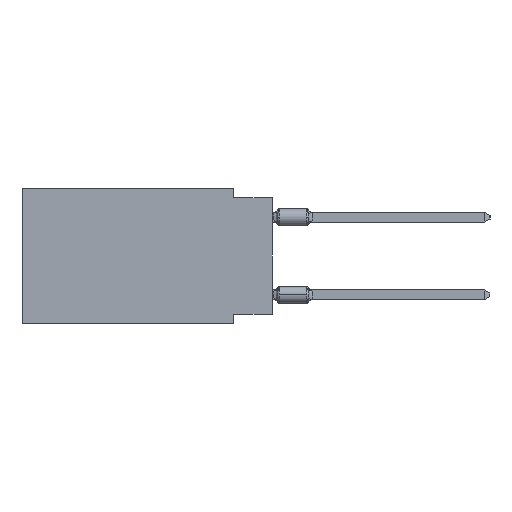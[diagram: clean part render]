
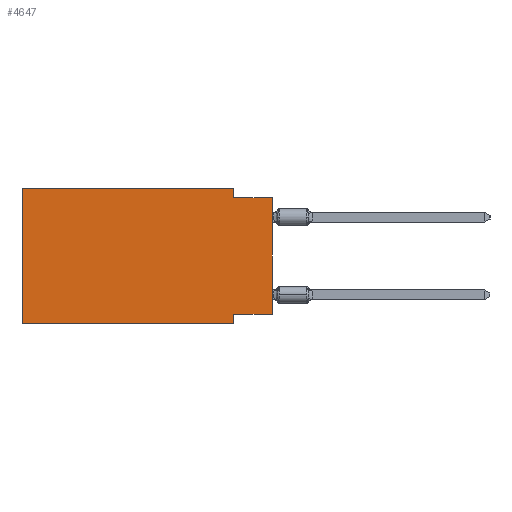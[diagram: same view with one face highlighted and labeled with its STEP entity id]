
A CAD part, left-side view. The second image highlights one B-rep face of the part: STEP entity #4647.
In plain terms, the highlighted planar face has unit normal (-1, 0, 0).
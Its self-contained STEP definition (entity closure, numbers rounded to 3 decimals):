
#118 = CARTESIAN_POINT ( 'NONE',  ( 0., 0., -0.635 ) ) ;
#2212 = EDGE_CURVE ( 'NONE', #31501, #4059, #9012, .T. ) ;
#2898 = ORIENTED_EDGE ( 'NONE', *, *, #9885, .F. ) ;
#3372 = LINE ( 'NONE', #16474, #13430 ) ;
#3487 = AXIS2_PLACEMENT_3D ( 'NONE', #16791, #22935, #10043 ) ;
#3642 = LINE ( 'NONE', #9602, #10874 ) ;
#3801 = VECTOR ( 'NONE', #16622, 1000. ) ;
#4059 = VERTEX_POINT ( 'NONE', #15455 ) ;
#4164 = DIRECTION ( 'NONE',  ( 0., -1., 0. ) ) ;
#4355 = CARTESIAN_POINT ( 'NONE',  ( 0., 16.383, 0. ) ) ;
#4647 = ADVANCED_FACE ( 'NONE', ( #23124 ), #10453, .F. ) ;
#5445 = CARTESIAN_POINT ( 'NONE',  ( 0., 0., -0.635 ) ) ;
#6313 = DIRECTION ( 'NONE',  ( 0., 0., -1. ) ) ;
#6758 = ORIENTED_EDGE ( 'NONE', *, *, #12679, .F. ) ;
#6772 = EDGE_LOOP ( 'NONE', ( #15858, #2898, #24143, #22416, #19249, #18441, #6758, #11832 ) ) ;
#6998 = VERTEX_POINT ( 'NONE', #19804 ) ;
#7661 = CARTESIAN_POINT ( 'NONE',  ( 0., 2.54, 0. ) ) ;
#7791 = VECTOR ( 'NONE', #22686, 1000. ) ;
#9012 = LINE ( 'NONE', #37650, #30920 ) ;
#9125 = LINE ( 'NONE', #12196, #16095 ) ;
#9602 = CARTESIAN_POINT ( 'NONE',  ( 0., 2.54, 0. ) ) ;
#9885 = EDGE_CURVE ( 'NONE', #39512, #22793, #27378, .T. ) ;
#10043 = DIRECTION ( 'NONE',  ( 0., 0., -1. ) ) ;
#10453 = PLANE ( 'NONE',  #3487 ) ;
#10716 = CARTESIAN_POINT ( 'NONE',  ( 0., 16.383, 0. ) ) ;
#10874 = VECTOR ( 'NONE', #6313, 1000. ) ;
#11756 = CARTESIAN_POINT ( 'NONE',  ( 0., 16.383, -8.89 ) ) ;
#11832 = ORIENTED_EDGE ( 'NONE', *, *, #13514, .F. ) ;
#12196 = CARTESIAN_POINT ( 'NONE',  ( 0., 16.383, 0. ) ) ;
#12679 = EDGE_CURVE ( 'NONE', #27653, #4059, #26644, .T. ) ;
#13430 = VECTOR ( 'NONE', #25894, 1000. ) ;
#13514 = EDGE_CURVE ( 'NONE', #6998, #27653, #32494, .T. ) ;
#15279 = DIRECTION ( 'NONE',  ( 0., -1., 0. ) ) ;
#15455 = CARTESIAN_POINT ( 'NONE',  ( 0., 2.54, -8.89 ) ) ;
#15858 = ORIENTED_EDGE ( 'NONE', *, *, #30050, .T. ) ;
#16095 = VECTOR ( 'NONE', #34294, 1000. ) ;
#16474 = CARTESIAN_POINT ( 'NONE',  ( 0., 0., 0. ) ) ;
#16622 = DIRECTION ( 'NONE',  ( 0., 0., -1. ) ) ;
#16791 = CARTESIAN_POINT ( 'NONE',  ( 0., 16.383, 0. ) ) ;
#16831 = CARTESIAN_POINT ( 'NONE',  ( 0., 2.54, -8.89 ) ) ;
#16938 = CARTESIAN_POINT ( 'NONE',  ( 0., 0., -8.255 ) ) ;
#18441 = ORIENTED_EDGE ( 'NONE', *, *, #2212, .T. ) ;
#18907 = CARTESIAN_POINT ( 'NONE',  ( 0., 2.54, -0.635 ) ) ;
#19249 = ORIENTED_EDGE ( 'NONE', *, *, #29057, .F. ) ;
#19594 = EDGE_CURVE ( 'NONE', #24459, #39439, #29148, .T. ) ;
#19804 = CARTESIAN_POINT ( 'NONE',  ( 0., 0., -8.255 ) ) ;
#21365 = CARTESIAN_POINT ( 'NONE',  ( 0., 2.54, -8.255 ) ) ;
#21511 = DIRECTION ( 'NONE',  ( 0., -1., 0. ) ) ;
#22416 = ORIENTED_EDGE ( 'NONE', *, *, #19594, .F. ) ;
#22686 = DIRECTION ( 'NONE',  ( 0., 1., 0. ) ) ;
#22793 = VERTEX_POINT ( 'NONE', #118 ) ;
#22935 = DIRECTION ( 'NONE',  ( 1., 0., 0. ) ) ;
#23124 = FACE_OUTER_BOUND ( 'NONE', #6772, .T. ) ;
#23600 = EDGE_CURVE ( 'NONE', #39439, #39512, #3642, .T. ) ;
#24143 = ORIENTED_EDGE ( 'NONE', *, *, #23600, .F. ) ;
#24459 = VERTEX_POINT ( 'NONE', #4355 ) ;
#25894 = DIRECTION ( 'NONE',  ( 0., 0., 1. ) ) ;
#26644 = LINE ( 'NONE', #16831, #3801 ) ;
#27378 = LINE ( 'NONE', #5445, #32557 ) ;
#27653 = VERTEX_POINT ( 'NONE', #21365 ) ;
#29057 = EDGE_CURVE ( 'NONE', #31501, #24459, #9125, .T. ) ;
#29148 = LINE ( 'NONE', #10716, #32288 ) ;
#30050 = EDGE_CURVE ( 'NONE', #6998, #22793, #3372, .T. ) ;
#30920 = VECTOR ( 'NONE', #21511, 1000. ) ;
#31501 = VERTEX_POINT ( 'NONE', #11756 ) ;
#32288 = VECTOR ( 'NONE', #4164, 1000. ) ;
#32494 = LINE ( 'NONE', #16938, #7791 ) ;
#32557 = VECTOR ( 'NONE', #15279, 1000. ) ;
#34294 = DIRECTION ( 'NONE',  ( 0., 0., 1. ) ) ;
#37650 = CARTESIAN_POINT ( 'NONE',  ( 0., 16.383, -8.89 ) ) ;
#39439 = VERTEX_POINT ( 'NONE', #7661 ) ;
#39512 = VERTEX_POINT ( 'NONE', #18907 ) ;
